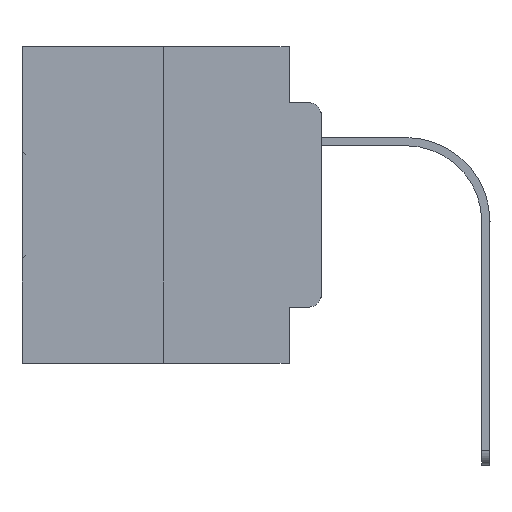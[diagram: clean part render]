
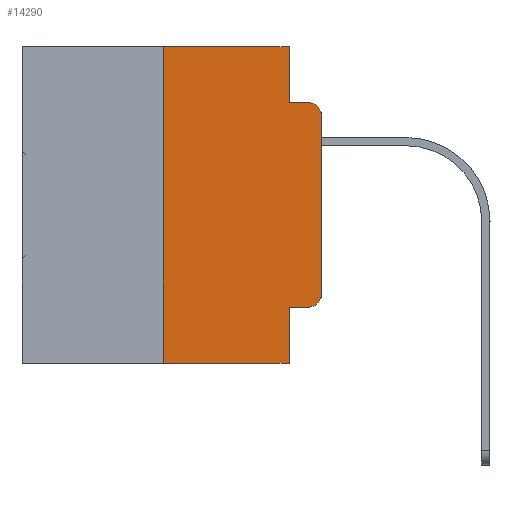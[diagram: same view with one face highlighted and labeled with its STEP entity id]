
A CAD part, left-side view. The second image highlights one B-rep face of the part: STEP entity #14290.
In plain terms, the highlighted planar face has unit normal (-1, 0, 0).
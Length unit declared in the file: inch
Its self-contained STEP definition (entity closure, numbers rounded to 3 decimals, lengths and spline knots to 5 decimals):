
#378 = EDGE_CURVE ( 'NONE', #30410, #22887, #7864, .T. ) ;
#395 = ORIENTED_EDGE ( 'NONE', *, *, #12736, .F. ) ;
#598 = CARTESIAN_POINT ( 'NONE',  ( 0., 0.473, 0. ) ) ;
#862 = DIRECTION ( 'NONE',  ( -1., 0., 0. ) ) ;
#1021 = CARTESIAN_POINT ( 'NONE',  ( 0., 0.02, -0.3915 ) ) ;
#1194 = FACE_OUTER_BOUND ( 'NONE', #28821, .T. ) ;
#1709 = CARTESIAN_POINT ( 'NONE',  ( 0., 0.25, 0. ) ) ;
#1775 = CIRCLE ( 'NONE', #11410, 0.02 ) ;
#1902 = CIRCLE ( 'NONE', #23709, 0.02 ) ;
#2489 = DIRECTION ( 'NONE',  ( 0., -1., 0. ) ) ;
#3111 = CARTESIAN_POINT ( 'NONE',  ( 0., 0.051, 0. ) ) ;
#3413 = DIRECTION ( 'NONE',  ( 0., 0., -1. ) ) ;
#3763 = VECTOR ( 'NONE', #2489, 39.37008 ) ;
#3766 = CARTESIAN_POINT ( 'NONE',  ( 0., 0.473, -0.5 ) ) ;
#5058 = LINE ( 'NONE', #598, #22303 ) ;
#5336 = DIRECTION ( 'NONE',  ( 0., 0., -1. ) ) ;
#5624 = EDGE_CURVE ( 'NONE', #15775, #22887, #13750, .T. ) ;
#5676 = DIRECTION ( 'NONE',  ( 0., -1., 0. ) ) ;
#6043 = EDGE_CURVE ( 'NONE', #10730, #17265, #28980, .T. ) ;
#6253 = CARTESIAN_POINT ( 'NONE',  ( 0., 0.02, -0.0885 ) ) ;
#6703 = ORIENTED_EDGE ( 'NONE', *, *, #5624, .T. ) ;
#6815 = ORIENTED_EDGE ( 'NONE', *, *, #7992, .T. ) ;
#7249 = LINE ( 'NONE', #22006, #3763 ) ;
#7864 = LINE ( 'NONE', #3111, #23220 ) ;
#7992 = EDGE_CURVE ( 'NONE', #17265, #10445, #1775, .T. ) ;
#8226 = VECTOR ( 'NONE', #14729, 39.37008 ) ;
#8390 = EDGE_CURVE ( 'NONE', #30410, #13547, #26361, .T. ) ;
#8910 = DIRECTION ( 'NONE',  ( -1., 0., 0. ) ) ;
#9350 = CARTESIAN_POINT ( 'NONE',  ( 0., 0.051, -0.4115 ) ) ;
#9876 = CARTESIAN_POINT ( 'NONE',  ( 0., 0.02, -0.4115 ) ) ;
#10158 = CARTESIAN_POINT ( 'NONE',  ( 0., 0.051, -0.0885 ) ) ;
#10221 = EDGE_CURVE ( 'NONE', #13547, #10730, #1902, .T. ) ;
#10445 = VERTEX_POINT ( 'NONE', #6253 ) ;
#10730 = VERTEX_POINT ( 'NONE', #23050 ) ;
#10890 = VECTOR ( 'NONE', #30387, 39.37008 ) ;
#11410 = AXIS2_PLACEMENT_3D ( 'NONE', #23841, #8910, #25598 ) ;
#11520 = CARTESIAN_POINT ( 'NONE',  ( 0., 0.051, 0. ) ) ;
#12219 = CARTESIAN_POINT ( 'NONE',  ( 0., 0.051, 0. ) ) ;
#12284 = CARTESIAN_POINT ( 'NONE',  ( 0., 0., 0. ) ) ;
#12376 = DIRECTION ( 'NONE',  ( 0., 0., -1. ) ) ;
#12736 = EDGE_CURVE ( 'NONE', #28553, #30768, #5058, .T. ) ;
#12754 = CARTESIAN_POINT ( 'NONE',  ( 0., 0.25, 0. ) ) ;
#13547 = VERTEX_POINT ( 'NONE', #9876 ) ;
#13750 = LINE ( 'NONE', #3766, #23662 ) ;
#13805 = VECTOR ( 'NONE', #12376, 39.37008 ) ;
#13925 = ORIENTED_EDGE ( 'NONE', *, *, #24133, .F. ) ;
#14043 = ORIENTED_EDGE ( 'NONE', *, *, #378, .F. ) ;
#14161 = ORIENTED_EDGE ( 'NONE', *, *, #8390, .T. ) ;
#14290 = ADVANCED_FACE ( 'NONE', ( #1194 ), #17528, .F. ) ;
#14729 = DIRECTION ( 'NONE',  ( 0., -1., 0. ) ) ;
#15775 = VERTEX_POINT ( 'NONE', #19560 ) ;
#16488 = ORIENTED_EDGE ( 'NONE', *, *, #24688, .F. ) ;
#17265 = VERTEX_POINT ( 'NONE', #20869 ) ;
#17528 = PLANE ( 'NONE',  #18531 ) ;
#17687 = CARTESIAN_POINT ( 'NONE',  ( 0., 0.473, 0. ) ) ;
#18354 = DIRECTION ( 'NONE',  ( 0., -1., 0. ) ) ;
#18531 = AXIS2_PLACEMENT_3D ( 'NONE', #17687, #24695, #3413 ) ;
#19560 = CARTESIAN_POINT ( 'NONE',  ( 0., 0.25, -0.5 ) ) ;
#19742 = DIRECTION ( 'NONE',  ( 0., 0., 1. ) ) ;
#20684 = LINE ( 'NONE', #12754, #10890 ) ;
#20869 = CARTESIAN_POINT ( 'NONE',  ( 0., 0., -0.1085 ) ) ;
#21751 = LINE ( 'NONE', #12219, #13805 ) ;
#22006 = CARTESIAN_POINT ( 'NONE',  ( 0., 0.051, -0.0885 ) ) ;
#22303 = VECTOR ( 'NONE', #5676, 39.37008 ) ;
#22887 = VERTEX_POINT ( 'NONE', #30628 ) ;
#23050 = CARTESIAN_POINT ( 'NONE',  ( 0., 0., -0.3915 ) ) ;
#23220 = VECTOR ( 'NONE', #5336, 39.37008 ) ;
#23639 = CARTESIAN_POINT ( 'NONE',  ( 0., 0.051, -0.4115 ) ) ;
#23662 = VECTOR ( 'NONE', #18354, 39.37008 ) ;
#23709 = AXIS2_PLACEMENT_3D ( 'NONE', #1021, #862, #30100 ) ;
#23841 = CARTESIAN_POINT ( 'NONE',  ( 0., 0.02, -0.1085 ) ) ;
#24133 = EDGE_CURVE ( 'NONE', #29589, #10445, #7249, .T. ) ;
#24688 = EDGE_CURVE ( 'NONE', #15775, #28553, #20684, .T. ) ;
#24695 = DIRECTION ( 'NONE',  ( 1., 0., 0. ) ) ;
#25598 = DIRECTION ( 'NONE',  ( 0., 0., -1. ) ) ;
#26361 = LINE ( 'NONE', #9350, #8226 ) ;
#26738 = ORIENTED_EDGE ( 'NONE', *, *, #6043, .T. ) ;
#27325 = ORIENTED_EDGE ( 'NONE', *, *, #10221, .T. ) ;
#28553 = VERTEX_POINT ( 'NONE', #1709 ) ;
#28821 = EDGE_LOOP ( 'NONE', ( #26738, #6815, #13925, #29912, #395, #16488, #6703, #14043, #14161, #27325 ) ) ;
#28980 = LINE ( 'NONE', #12284, #29570 ) ;
#29417 = EDGE_CURVE ( 'NONE', #30768, #29589, #21751, .T. ) ;
#29570 = VECTOR ( 'NONE', #19742, 39.37008 ) ;
#29589 = VERTEX_POINT ( 'NONE', #10158 ) ;
#29912 = ORIENTED_EDGE ( 'NONE', *, *, #29417, .F. ) ;
#30100 = DIRECTION ( 'NONE',  ( 0., 0., -1. ) ) ;
#30387 = DIRECTION ( 'NONE',  ( 0., 0., 1. ) ) ;
#30410 = VERTEX_POINT ( 'NONE', #23639 ) ;
#30628 = CARTESIAN_POINT ( 'NONE',  ( 0., 0.051, -0.5 ) ) ;
#30768 = VERTEX_POINT ( 'NONE', #11520 ) ;
